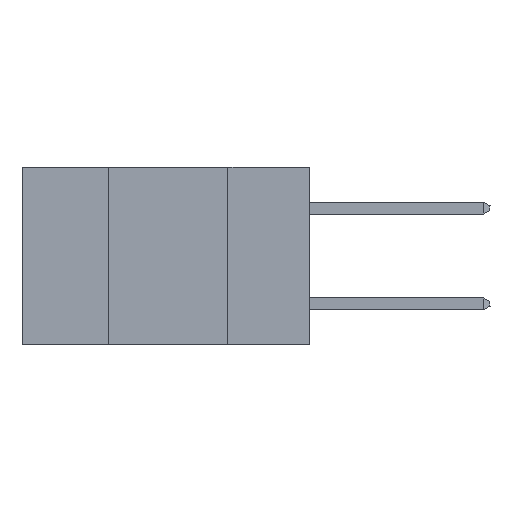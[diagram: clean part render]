
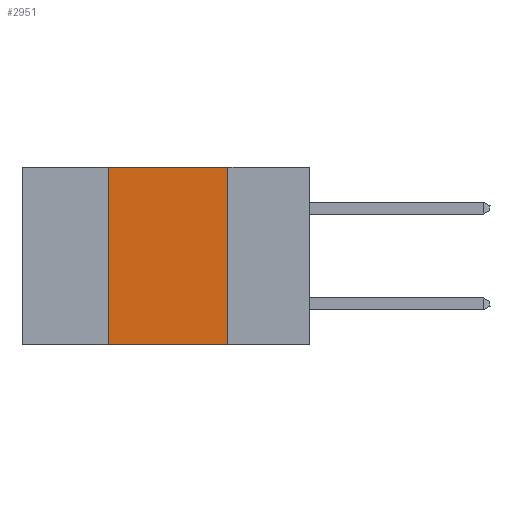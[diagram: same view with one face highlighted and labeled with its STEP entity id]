
A CAD part, left-side view. The second image highlights one B-rep face of the part: STEP entity #2951.
In plain terms, the highlighted planar face has unit normal (-1, 0, 0).
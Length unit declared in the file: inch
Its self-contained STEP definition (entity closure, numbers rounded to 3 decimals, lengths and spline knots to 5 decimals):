
#348 = LINE ( 'NONE', #19066, #9451 ) ;
#718 = DIRECTION ( 'NONE',  ( 0., 0., 1. ) ) ;
#1127 = EDGE_CURVE ( 'NONE', #20941, #22852, #16702, .T. ) ;
#2951 = ADVANCED_FACE ( 'NONE', ( #11208 ), #26333, .F. ) ;
#3409 = ORIENTED_EDGE ( 'NONE', *, *, #1127, .F. ) ;
#3592 = VERTEX_POINT ( 'NONE', #5977 ) ;
#5977 = CARTESIAN_POINT ( 'NONE',  ( 0., 0.42, 0. ) ) ;
#6249 = DIRECTION ( 'NONE',  ( 0., 0., -1. ) ) ;
#8475 = ORIENTED_EDGE ( 'NONE', *, *, #19725, .T. ) ;
#8900 = EDGE_CURVE ( 'NONE', #10474, #3592, #15833, .T. ) ;
#9451 = VECTOR ( 'NONE', #16648, 39.37008 ) ;
#9481 = ORIENTED_EDGE ( 'NONE', *, *, #25625, .F. ) ;
#10474 = VERTEX_POINT ( 'NONE', #17148 ) ;
#10994 = VECTOR ( 'NONE', #21456, 39.37008 ) ;
#11208 = FACE_OUTER_BOUND ( 'NONE', #23746, .T. ) ;
#12424 = VECTOR ( 'NONE', #17336, 39.37008 ) ;
#13790 = ORIENTED_EDGE ( 'NONE', *, *, #8900, .F. ) ;
#15267 = CARTESIAN_POINT ( 'NONE',  ( 0., 0.6, 0. ) ) ;
#15828 = CARTESIAN_POINT ( 'NONE',  ( 0., 0.42, 0. ) ) ;
#15833 = LINE ( 'NONE', #15828, #25576 ) ;
#16648 = DIRECTION ( 'NONE',  ( 0., -1., 0. ) ) ;
#16702 = LINE ( 'NONE', #25790, #10994 ) ;
#16917 = AXIS2_PLACEMENT_3D ( 'NONE', #21429, #21253, #6249 ) ;
#17148 = CARTESIAN_POINT ( 'NONE',  ( 0., 0.42, -0.37 ) ) ;
#17336 = DIRECTION ( 'NONE',  ( 0., -1., 0. ) ) ;
#17909 = LINE ( 'NONE', #15267, #12424 ) ;
#19066 = CARTESIAN_POINT ( 'NONE',  ( 0., 0.6, -0.37 ) ) ;
#19725 = EDGE_CURVE ( 'NONE', #10474, #22852, #348, .T. ) ;
#20941 = VERTEX_POINT ( 'NONE', #23233 ) ;
#21253 = DIRECTION ( 'NONE',  ( 1., 0., 0. ) ) ;
#21429 = CARTESIAN_POINT ( 'NONE',  ( 0., 0.6, 0. ) ) ;
#21456 = DIRECTION ( 'NONE',  ( 0., 0., -1. ) ) ;
#22852 = VERTEX_POINT ( 'NONE', #25541 ) ;
#23233 = CARTESIAN_POINT ( 'NONE',  ( 0., 0.17, 0. ) ) ;
#23746 = EDGE_LOOP ( 'NONE', ( #3409, #9481, #13790, #8475 ) ) ;
#25541 = CARTESIAN_POINT ( 'NONE',  ( 0., 0.17, -0.37 ) ) ;
#25576 = VECTOR ( 'NONE', #718, 39.37008 ) ;
#25625 = EDGE_CURVE ( 'NONE', #3592, #20941, #17909, .T. ) ;
#25790 = CARTESIAN_POINT ( 'NONE',  ( 0., 0.17, 0. ) ) ;
#26333 = PLANE ( 'NONE',  #16917 ) ;
